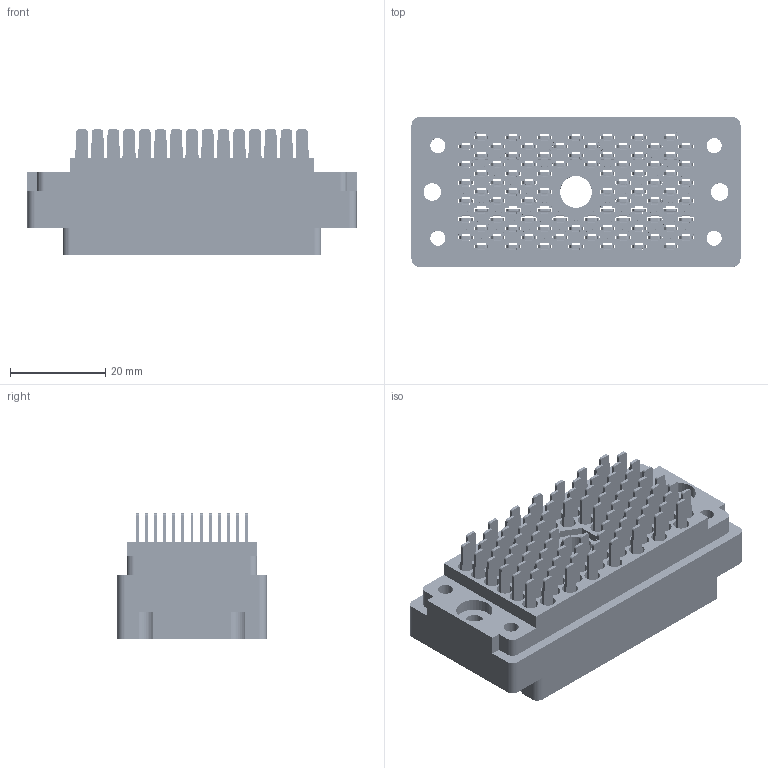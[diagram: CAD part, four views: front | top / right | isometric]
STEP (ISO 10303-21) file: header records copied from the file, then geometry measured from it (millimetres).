
FILE_DESCRIPTION (( 'STEP AP203' ), '1' );
FILE_NAME ('516-090-501-300.STEP', '2020-09-08T06:33:08', ( '' ), ( '' ), 'SwSTEP 2.0', 'SolidWorks 2020', '' );
FILE_SCHEMA (( 'CONFIG_CONTROL_DESIGN' ));
Length unit declared in the file: inch
Products named in the file (3): 516 Plug Insulator_090; 516-090-501-300; 516-292-001_501 Contact
Assembly tree (91 placements, depth 2):
  516-090-501-300
    516 Plug Insulator_090
    516-292-001_501 Contact  x90
Bounding box: 69.04 x 31.34 x 26.26 mm (x, y, z)
Volume: 20367.1 mm3; surface area: 38911.7 mm2
Topology: 91 solids, 91 shells, 8326 faces, 24212 edges, 16080 vertices
Faces by surface type: plane 5073, cylinder 2711, bspline 540, cone 2
Entity records: 67950 total; most frequent: CARTESIAN_POINT 11795, ORIENTED_EDGE 11400, DIRECTION 11010, EDGE_CURVE 5700, LINE 4334, VECTOR 4334, VERTEX_POINT 3798, AXIS2_PLACEMENT_3D 3338
